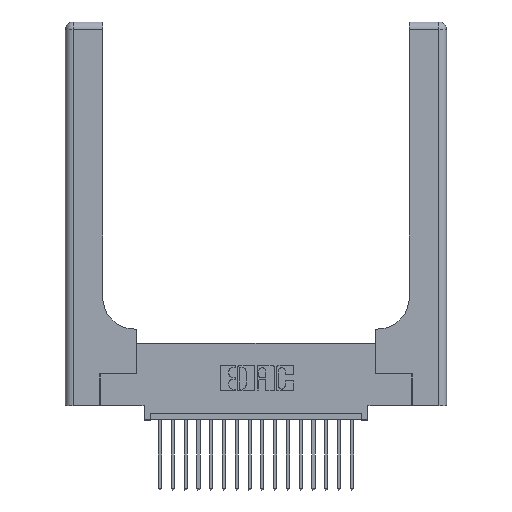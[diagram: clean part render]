
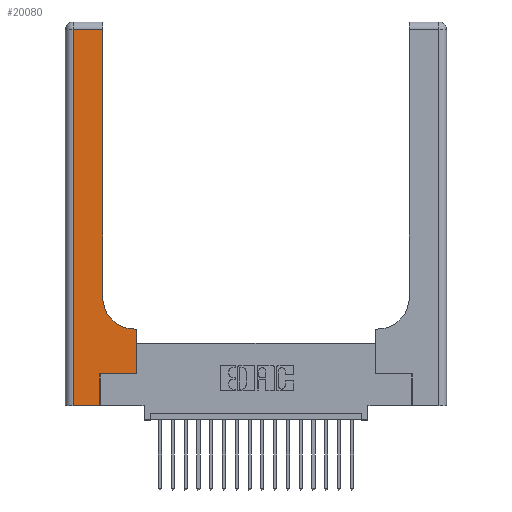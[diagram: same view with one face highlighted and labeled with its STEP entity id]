
A CAD part, top view. The second image highlights one B-rep face of the part: STEP entity #20080.
In plain terms, the highlighted planar face has unit normal (0, 0, 1).
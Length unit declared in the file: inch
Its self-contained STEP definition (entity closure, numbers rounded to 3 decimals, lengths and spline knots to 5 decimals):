
#23 = VERTEX_POINT ( 'NONE', #18265 ) ;
#550 = EDGE_CURVE ( 'NONE', #19340, #18703, #3562, .T. ) ;
#612 = DIRECTION ( 'NONE',  ( 0., -1., 0. ) ) ;
#761 = DIRECTION ( 'NONE',  ( 1., 0., 0. ) ) ;
#1333 = ORIENTED_EDGE ( 'NONE', *, *, #18939, .T. ) ;
#1487 = VERTEX_POINT ( 'NONE', #11740 ) ;
#1563 = CARTESIAN_POINT ( 'NONE',  ( 0.5585, 0.25, 0.37 ) ) ;
#2132 = VERTEX_POINT ( 'NONE', #9362 ) ;
#2160 = CARTESIAN_POINT ( 'NONE',  ( 0.269, 0., 0.37 ) ) ;
#2261 = ORIENTED_EDGE ( 'NONE', *, *, #550, .T. ) ;
#2391 = CARTESIAN_POINT ( 'NONE',  ( 0.06, 2.94, 0.37 ) ) ;
#2518 = VECTOR ( 'NONE', #19317, 39.37008 ) ;
#2645 = FACE_OUTER_BOUND ( 'NONE', #17319, .T. ) ;
#2654 = DIRECTION ( 'NONE',  ( 0., 1., 0. ) ) ;
#2939 = ORIENTED_EDGE ( 'NONE', *, *, #8083, .T. ) ;
#3238 = VERTEX_POINT ( 'NONE', #17419 ) ;
#3507 = CARTESIAN_POINT ( 'NONE',  ( 0.5585, 0.25, 0.37 ) ) ;
#3562 = LINE ( 'NONE', #4890, #12136 ) ;
#3665 = EDGE_CURVE ( 'NONE', #6167, #6430, #6990, .T. ) ;
#4015 = CARTESIAN_POINT ( 'NONE',  ( 0.269, 0.25, 0.37 ) ) ;
#4046 = LINE ( 'NONE', #14483, #2518 ) ;
#4182 = LINE ( 'NONE', #8105, #12252 ) ;
#4890 = CARTESIAN_POINT ( 'NONE',  ( 0., 0., 0.37 ) ) ;
#5282 = CARTESIAN_POINT ( 'NONE',  ( 0.06, 3., 0.37 ) ) ;
#5730 = CARTESIAN_POINT ( 'NONE',  ( 0.269, 0., 0.37 ) ) ;
#5895 = ORIENTED_EDGE ( 'NONE', *, *, #17928, .T. ) ;
#6167 = VERTEX_POINT ( 'NONE', #15771 ) ;
#6429 = PLANE ( 'NONE',  #11417 ) ;
#6430 = VERTEX_POINT ( 'NONE', #1563 ) ;
#6537 = ORIENTED_EDGE ( 'NONE', *, *, #10295, .T. ) ;
#6758 = VERTEX_POINT ( 'NONE', #2391 ) ;
#6990 = LINE ( 'NONE', #4015, #19359 ) ;
#7000 = LINE ( 'NONE', #2160, #9248 ) ;
#7185 = DIRECTION ( 'NONE',  ( 1., 0., 0. ) ) ;
#7337 = CARTESIAN_POINT ( 'NONE',  ( 0.06, 0., 0.37 ) ) ;
#7675 = VECTOR ( 'NONE', #2654, 39.37008 ) ;
#8083 = EDGE_CURVE ( 'NONE', #6758, #19340, #9594, .T. ) ;
#8105 = CARTESIAN_POINT ( 'NONE',  ( 0., 2.94, 0.37 ) ) ;
#8554 = AXIS2_PLACEMENT_3D ( 'NONE', #13632, #19911, #761 ) ;
#8566 = VECTOR ( 'NONE', #612, 39.37008 ) ;
#8640 = LINE ( 'NONE', #3507, #10412 ) ;
#9248 = VECTOR ( 'NONE', #16589, 39.37008 ) ;
#9362 = CARTESIAN_POINT ( 'NONE',  ( 0.5415, 0.6, 0.37 ) ) ;
#9594 = LINE ( 'NONE', #5282, #8566 ) ;
#9639 = DIRECTION ( 'NONE',  ( 0., 1., 0. ) ) ;
#10295 = EDGE_CURVE ( 'NONE', #6430, #23, #8640, .T. ) ;
#10412 = VECTOR ( 'NONE', #9639, 39.37008 ) ;
#11136 = DIRECTION ( 'NONE',  ( 0., 0., -1. ) ) ;
#11417 = AXIS2_PLACEMENT_3D ( 'NONE', #20794, #11136, #15962 ) ;
#11740 = CARTESIAN_POINT ( 'NONE',  ( 0.2915, 2.94, 0.37 ) ) ;
#11877 = ORIENTED_EDGE ( 'NONE', *, *, #20314, .T. ) ;
#11906 = EDGE_CURVE ( 'NONE', #23, #2132, #4046, .T. ) ;
#12136 = VECTOR ( 'NONE', #12925, 39.37008 ) ;
#12252 = VECTOR ( 'NONE', #16054, 39.37008 ) ;
#12311 = CARTESIAN_POINT ( 'NONE',  ( 0.2915, 3., 0.37 ) ) ;
#12925 = DIRECTION ( 'NONE',  ( 1., 0., 0. ) ) ;
#13632 = CARTESIAN_POINT ( 'NONE',  ( 0.5415, 0.85, 0.37 ) ) ;
#14483 = CARTESIAN_POINT ( 'NONE',  ( 0.2915, 0.6, 0.37 ) ) ;
#14693 = ORIENTED_EDGE ( 'NONE', *, *, #11906, .T. ) ;
#15771 = CARTESIAN_POINT ( 'NONE',  ( 0.269, 0.25, 0.37 ) ) ;
#15853 = ORIENTED_EDGE ( 'NONE', *, *, #19811, .T. ) ;
#15962 = DIRECTION ( 'NONE',  ( -1., 0., 0. ) ) ;
#16054 = DIRECTION ( 'NONE',  ( -1., 0., 0. ) ) ;
#16448 = ORIENTED_EDGE ( 'NONE', *, *, #3665, .T. ) ;
#16589 = DIRECTION ( 'NONE',  ( 0., 1., 0. ) ) ;
#17029 = LINE ( 'NONE', #12311, #7675 ) ;
#17265 = CIRCLE ( 'NONE', #8554, 0.25 ) ;
#17319 = EDGE_LOOP ( 'NONE', ( #11877, #1333, #2939, #2261, #5895, #16448, #6537, #14693, #15853 ) ) ;
#17419 = CARTESIAN_POINT ( 'NONE',  ( 0.2915, 0.85, 0.37 ) ) ;
#17928 = EDGE_CURVE ( 'NONE', #18703, #6167, #7000, .T. ) ;
#18265 = CARTESIAN_POINT ( 'NONE',  ( 0.5585, 0.6, 0.37 ) ) ;
#18703 = VERTEX_POINT ( 'NONE', #5730 ) ;
#18939 = EDGE_CURVE ( 'NONE', #1487, #6758, #4182, .T. ) ;
#19317 = DIRECTION ( 'NONE',  ( -1., 0., 0. ) ) ;
#19340 = VERTEX_POINT ( 'NONE', #7337 ) ;
#19359 = VECTOR ( 'NONE', #7185, 39.37008 ) ;
#19811 = EDGE_CURVE ( 'NONE', #2132, #3238, #17265, .T. ) ;
#19911 = DIRECTION ( 'NONE',  ( 0., 0., -1. ) ) ;
#20080 = ADVANCED_FACE ( 'NONE', ( #2645 ), #6429, .F. ) ;
#20314 = EDGE_CURVE ( 'NONE', #3238, #1487, #17029, .T. ) ;
#20794 = CARTESIAN_POINT ( 'NONE',  ( 0., 3., 0.37 ) ) ;
